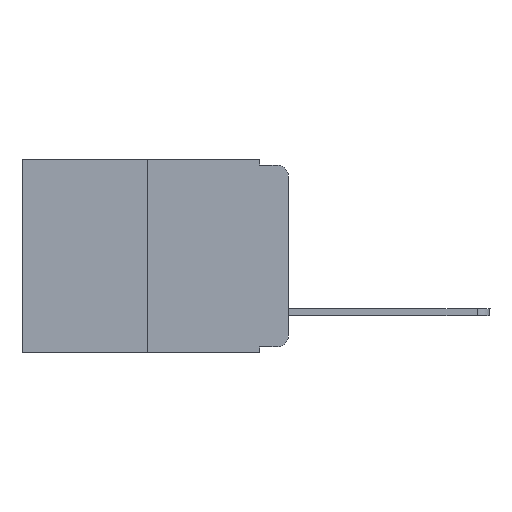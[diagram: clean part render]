
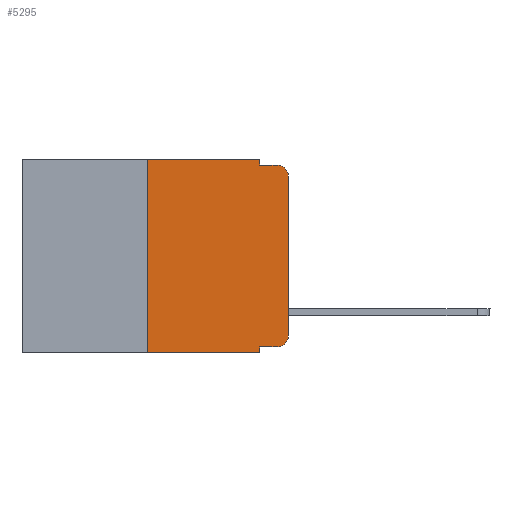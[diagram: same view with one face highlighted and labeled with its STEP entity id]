
A CAD part, left-side view. The second image highlights one B-rep face of the part: STEP entity #5295.
In plain terms, the highlighted planar face has unit normal (-1, 0, 0).
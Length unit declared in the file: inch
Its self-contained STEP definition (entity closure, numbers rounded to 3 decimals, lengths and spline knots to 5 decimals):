
#222 = DIRECTION ( 'NONE',  ( 0., -1., 0. ) ) ;
#472 = ORIENTED_EDGE ( 'NONE', *, *, #7602, .F. ) ;
#641 = CARTESIAN_POINT ( 'NONE',  ( 0., 0.051, 0. ) ) ;
#996 = DIRECTION ( 'NONE',  ( 0., 0., -1. ) ) ;
#1258 = VECTOR ( 'NONE', #14019, 39.37008 ) ;
#1555 = CIRCLE ( 'NONE', #14916, 0.02 ) ;
#1869 = VERTEX_POINT ( 'NONE', #3488 ) ;
#2087 = EDGE_CURVE ( 'NONE', #6636, #10582, #4236, .T. ) ;
#2182 = DIRECTION ( 'NONE',  ( 0., 0., -1. ) ) ;
#2290 = VERTEX_POINT ( 'NONE', #7224 ) ;
#2317 = AXIS2_PLACEMENT_3D ( 'NONE', #11236, #15249, #7219 ) ;
#2866 = CARTESIAN_POINT ( 'NONE',  ( 0., 0.051, -0.333 ) ) ;
#3266 = ORIENTED_EDGE ( 'NONE', *, *, #3654, .F. ) ;
#3488 = CARTESIAN_POINT ( 'NONE',  ( 0., 0.051, -0.01 ) ) ;
#3502 = ORIENTED_EDGE ( 'NONE', *, *, #15891, .F. ) ;
#3516 = VECTOR ( 'NONE', #12015, 39.37008 ) ;
#3624 = DIRECTION ( 'NONE',  ( -1., 0., 0. ) ) ;
#3654 = EDGE_CURVE ( 'NONE', #10740, #1869, #8690, .T. ) ;
#3800 = ORIENTED_EDGE ( 'NONE', *, *, #5716, .T. ) ;
#4052 = CARTESIAN_POINT ( 'NONE',  ( 0., 0., -0.03 ) ) ;
#4236 = LINE ( 'NONE', #12105, #11674 ) ;
#4389 = VERTEX_POINT ( 'NONE', #11896 ) ;
#4625 = EDGE_CURVE ( 'NONE', #12650, #10582, #12659, .T. ) ;
#4753 = VERTEX_POINT ( 'NONE', #6750 ) ;
#4817 = LINE ( 'NONE', #11409, #10793 ) ;
#5295 = ADVANCED_FACE ( 'NONE', ( #8608 ), #7492, .F. ) ;
#5334 = ORIENTED_EDGE ( 'NONE', *, *, #6888, .T. ) ;
#5396 = DIRECTION ( 'NONE',  ( 0., -1., 0. ) ) ;
#5514 = VECTOR ( 'NONE', #7398, 39.37008 ) ;
#5716 = EDGE_CURVE ( 'NONE', #2290, #4753, #10805, .T. ) ;
#5951 = ORIENTED_EDGE ( 'NONE', *, *, #4625, .F. ) ;
#6204 = DIRECTION ( 'NONE',  ( 0., 0., 1. ) ) ;
#6559 = ORIENTED_EDGE ( 'NONE', *, *, #13592, .T. ) ;
#6636 = VERTEX_POINT ( 'NONE', #14312 ) ;
#6705 = DIRECTION ( 'NONE',  ( 0., 0., 1. ) ) ;
#6750 = CARTESIAN_POINT ( 'NONE',  ( 0., 0., -0.313 ) ) ;
#6888 = EDGE_CURVE ( 'NONE', #4753, #13849, #4817, .T. ) ;
#6985 = VERTEX_POINT ( 'NONE', #7139 ) ;
#7139 = CARTESIAN_POINT ( 'NONE',  ( 0., 0.25, 0. ) ) ;
#7219 = DIRECTION ( 'NONE',  ( 0., 0., -1. ) ) ;
#7224 = CARTESIAN_POINT ( 'NONE',  ( 0., 0.02, -0.333 ) ) ;
#7398 = DIRECTION ( 'NONE',  ( 0., 0., -1. ) ) ;
#7492 = PLANE ( 'NONE',  #15172 ) ;
#7602 = EDGE_CURVE ( 'NONE', #6985, #10740, #14610, .T. ) ;
#7688 = ORIENTED_EDGE ( 'NONE', *, *, #16367, .F. ) ;
#7874 = ORIENTED_EDGE ( 'NONE', *, *, #15047, .T. ) ;
#8413 = VECTOR ( 'NONE', #6705, 39.37008 ) ;
#8608 = FACE_OUTER_BOUND ( 'NONE', #15793, .T. ) ;
#8635 = DIRECTION ( 'NONE',  ( 0., -1., 0. ) ) ;
#8690 = LINE ( 'NONE', #641, #5514 ) ;
#9385 = LINE ( 'NONE', #2866, #3516 ) ;
#9781 = VECTOR ( 'NONE', #8635, 39.37008 ) ;
#10397 = CARTESIAN_POINT ( 'NONE',  ( 0., 0.25, 0. ) ) ;
#10582 = VERTEX_POINT ( 'NONE', #15876 ) ;
#10740 = VERTEX_POINT ( 'NONE', #16370 ) ;
#10793 = VECTOR ( 'NONE', #6204, 39.37008 ) ;
#10805 = CIRCLE ( 'NONE', #2317, 0.02 ) ;
#11236 = CARTESIAN_POINT ( 'NONE',  ( 0., 0.02, -0.313 ) ) ;
#11334 = CARTESIAN_POINT ( 'NONE',  ( 0., 0.473, 0. ) ) ;
#11409 = CARTESIAN_POINT ( 'NONE',  ( 0., 0., 0. ) ) ;
#11674 = VECTOR ( 'NONE', #222, 39.37008 ) ;
#11838 = LINE ( 'NONE', #10397, #8413 ) ;
#11891 = CARTESIAN_POINT ( 'NONE',  ( 0., 0.473, 0. ) ) ;
#11896 = CARTESIAN_POINT ( 'NONE',  ( 0., 0.02, -0.01 ) ) ;
#12015 = DIRECTION ( 'NONE',  ( 0., -1., 0. ) ) ;
#12105 = CARTESIAN_POINT ( 'NONE',  ( 0., 0.473, -0.343 ) ) ;
#12393 = LINE ( 'NONE', #16232, #9781 ) ;
#12650 = VERTEX_POINT ( 'NONE', #13965 ) ;
#12659 = LINE ( 'NONE', #15382, #1258 ) ;
#13592 = EDGE_CURVE ( 'NONE', #12650, #2290, #9385, .T. ) ;
#13849 = VERTEX_POINT ( 'NONE', #4052 ) ;
#13896 = CARTESIAN_POINT ( 'NONE',  ( 0., 0.02, -0.03 ) ) ;
#13965 = CARTESIAN_POINT ( 'NONE',  ( 0., 0.051, -0.333 ) ) ;
#14019 = DIRECTION ( 'NONE',  ( 0., 0., -1. ) ) ;
#14312 = CARTESIAN_POINT ( 'NONE',  ( 0., 0.25, -0.343 ) ) ;
#14610 = LINE ( 'NONE', #11891, #14642 ) ;
#14642 = VECTOR ( 'NONE', #5396, 39.37008 ) ;
#14916 = AXIS2_PLACEMENT_3D ( 'NONE', #13896, #3624, #2182 ) ;
#15047 = EDGE_CURVE ( 'NONE', #13849, #4389, #1555, .T. ) ;
#15172 = AXIS2_PLACEMENT_3D ( 'NONE', #11334, #16545, #996 ) ;
#15249 = DIRECTION ( 'NONE',  ( -1., 0., 0. ) ) ;
#15382 = CARTESIAN_POINT ( 'NONE',  ( 0., 0.051, 0. ) ) ;
#15637 = ORIENTED_EDGE ( 'NONE', *, *, #2087, .T. ) ;
#15793 = EDGE_LOOP ( 'NONE', ( #5334, #7874, #3502, #3266, #472, #7688, #15637, #5951, #6559, #3800 ) ) ;
#15876 = CARTESIAN_POINT ( 'NONE',  ( 0., 0.051, -0.343 ) ) ;
#15891 = EDGE_CURVE ( 'NONE', #1869, #4389, #12393, .T. ) ;
#16232 = CARTESIAN_POINT ( 'NONE',  ( 0., 0.051, -0.01 ) ) ;
#16367 = EDGE_CURVE ( 'NONE', #6636, #6985, #11838, .T. ) ;
#16370 = CARTESIAN_POINT ( 'NONE',  ( 0., 0.051, 0. ) ) ;
#16545 = DIRECTION ( 'NONE',  ( 1., 0., 0. ) ) ;
